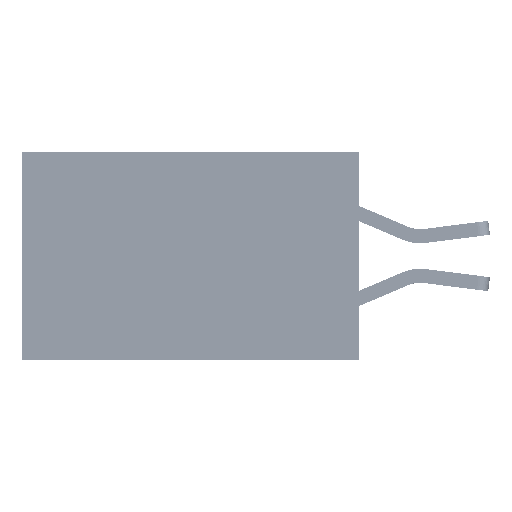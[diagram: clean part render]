
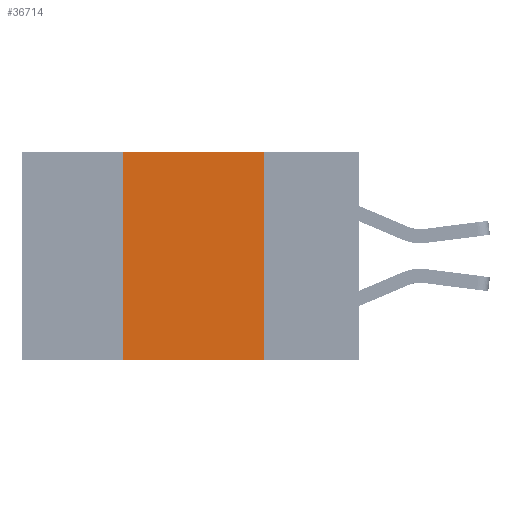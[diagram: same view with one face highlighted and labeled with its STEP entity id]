
A CAD part, left-side view. The second image highlights one B-rep face of the part: STEP entity #36714.
In plain terms, the highlighted planar face has unit normal (-1, 0, 0).
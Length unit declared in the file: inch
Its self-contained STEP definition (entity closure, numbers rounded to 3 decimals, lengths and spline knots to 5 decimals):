
#221 = LINE ( 'NONE', #14717, #43392 ) ;
#1515 = DIRECTION ( 'NONE',  ( 0., -1., 0. ) ) ;
#2922 = EDGE_CURVE ( 'NONE', #42910, #22511, #221, .T. ) ;
#4373 = VERTEX_POINT ( 'NONE', #10511 ) ;
#6994 = DIRECTION ( 'NONE',  ( 0., 0., 1. ) ) ;
#10511 = CARTESIAN_POINT ( 'NONE',  ( 0., 0.17, -0.37 ) ) ;
#11282 = LINE ( 'NONE', #39139, #20387 ) ;
#12371 = EDGE_CURVE ( 'NONE', #22511, #35704, #41241, .T. ) ;
#12474 = CARTESIAN_POINT ( 'NONE',  ( 0., 0.6, 0. ) ) ;
#13067 = ORIENTED_EDGE ( 'NONE', *, *, #12371, .F. ) ;
#14717 = CARTESIAN_POINT ( 'NONE',  ( 0., 0.42, 0. ) ) ;
#15026 = DIRECTION ( 'NONE',  ( 1., 0., 0. ) ) ;
#15496 = FACE_OUTER_BOUND ( 'NONE', #19756, .T. ) ;
#15559 = LINE ( 'NONE', #19542, #31708 ) ;
#15681 = VECTOR ( 'NONE', #15983, 39.37008 ) ;
#15983 = DIRECTION ( 'NONE',  ( 0., -1., 0. ) ) ;
#18703 = CARTESIAN_POINT ( 'NONE',  ( 0., 0.17, 0. ) ) ;
#19542 = CARTESIAN_POINT ( 'NONE',  ( 0., 0.6, -0.37 ) ) ;
#19756 = EDGE_LOOP ( 'NONE', ( #20437, #13067, #30559, #22809 ) ) ;
#20387 = VECTOR ( 'NONE', #31898, 39.37008 ) ;
#20437 = ORIENTED_EDGE ( 'NONE', *, *, #44323, .F. ) ;
#22511 = VERTEX_POINT ( 'NONE', #39577 ) ;
#22809 = ORIENTED_EDGE ( 'NONE', *, *, #33146, .T. ) ;
#27813 = CARTESIAN_POINT ( 'NONE',  ( 0., 0.42, -0.37 ) ) ;
#30559 = ORIENTED_EDGE ( 'NONE', *, *, #2922, .F. ) ;
#31708 = VECTOR ( 'NONE', #1515, 39.37008 ) ;
#31898 = DIRECTION ( 'NONE',  ( 0., 0., -1. ) ) ;
#32345 = CARTESIAN_POINT ( 'NONE',  ( 0., 0.6, 0. ) ) ;
#33146 = EDGE_CURVE ( 'NONE', #42910, #4373, #15559, .T. ) ;
#35704 = VERTEX_POINT ( 'NONE', #18703 ) ;
#36714 = ADVANCED_FACE ( 'NONE', ( #15496 ), #43326, .F. ) ;
#38729 = DIRECTION ( 'NONE',  ( 0., 0., -1. ) ) ;
#39139 = CARTESIAN_POINT ( 'NONE',  ( 0., 0.17, 0. ) ) ;
#39577 = CARTESIAN_POINT ( 'NONE',  ( 0., 0.42, 0. ) ) ;
#41241 = LINE ( 'NONE', #12474, #15681 ) ;
#41840 = AXIS2_PLACEMENT_3D ( 'NONE', #32345, #15026, #38729 ) ;
#42910 = VERTEX_POINT ( 'NONE', #27813 ) ;
#43326 = PLANE ( 'NONE',  #41840 ) ;
#43392 = VECTOR ( 'NONE', #6994, 39.37008 ) ;
#44323 = EDGE_CURVE ( 'NONE', #35704, #4373, #11282, .T. ) ;
